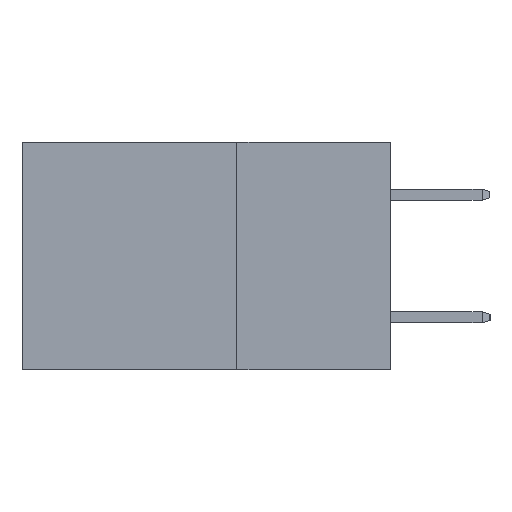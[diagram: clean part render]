
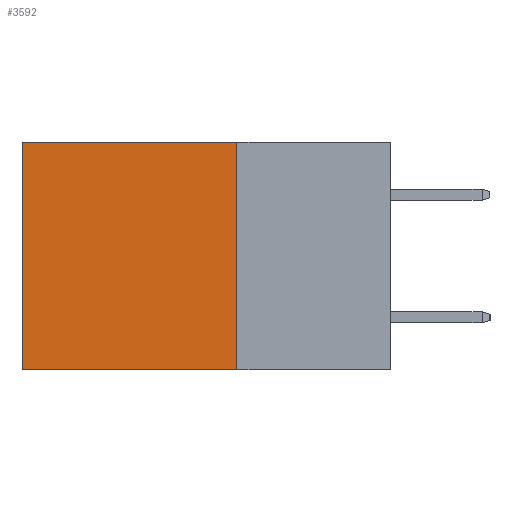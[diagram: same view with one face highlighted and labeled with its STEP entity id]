
A CAD part, left-side view. The second image highlights one B-rep face of the part: STEP entity #3592.
In plain terms, the highlighted planar face has unit normal (-1, 0, 0).
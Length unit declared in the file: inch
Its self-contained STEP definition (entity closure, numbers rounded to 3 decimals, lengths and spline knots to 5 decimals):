
#860 = ORIENTED_EDGE ( 'NONE', *, *, #4558, .F. ) ;
#1102 = VERTEX_POINT ( 'NONE', #10392 ) ;
#1399 = DIRECTION ( 'NONE',  ( 0., 0., -1. ) ) ;
#1477 = VERTEX_POINT ( 'NONE', #8669 ) ;
#1586 = ORIENTED_EDGE ( 'NONE', *, *, #10714, .T. ) ;
#1607 = VERTEX_POINT ( 'NONE', #12531 ) ;
#2351 = DIRECTION ( 'NONE',  ( 1., 0., 0. ) ) ;
#2871 = ORIENTED_EDGE ( 'NONE', *, *, #3994, .T. ) ;
#3326 = CARTESIAN_POINT ( 'NONE',  ( 0.2875, 0.25, 0. ) ) ;
#3592 = ADVANCED_FACE ( 'NONE', ( #5647 ), #9810, .F. ) ;
#3950 = LINE ( 'NONE', #3326, #10380 ) ;
#3994 = EDGE_CURVE ( 'NONE', #1607, #1477, #13299, .T. ) ;
#4436 = LINE ( 'NONE', #9249, #7094 ) ;
#4558 = EDGE_CURVE ( 'NONE', #1102, #9808, #4436, .T. ) ;
#5647 = FACE_OUTER_BOUND ( 'NONE', #9036, .T. ) ;
#7094 = VECTOR ( 'NONE', #1399, 39.37008 ) ;
#8139 = CARTESIAN_POINT ( 'NONE',  ( 0.2875, 0.25, -0.37 ) ) ;
#8602 = CARTESIAN_POINT ( 'NONE',  ( 0.2875, 0.25, 0. ) ) ;
#8669 = CARTESIAN_POINT ( 'NONE',  ( 0.2875, 0.6, -0.37 ) ) ;
#8884 = DIRECTION ( 'NONE',  ( 0., 0., -1. ) ) ;
#9036 = EDGE_LOOP ( 'NONE', ( #2871, #10672, #860, #1586 ) ) ;
#9249 = CARTESIAN_POINT ( 'NONE',  ( 0.2875, 0.25, 0. ) ) ;
#9670 = DIRECTION ( 'NONE',  ( 0., 1., 0. ) ) ;
#9713 = AXIS2_PLACEMENT_3D ( 'NONE', #8602, #2351, #12806 ) ;
#9808 = VERTEX_POINT ( 'NONE', #8139 ) ;
#9810 = PLANE ( 'NONE',  #9713 ) ;
#10051 = CARTESIAN_POINT ( 'NONE',  ( 0.2875, 0.25, -0.37 ) ) ;
#10380 = VECTOR ( 'NONE', #9670, 39.37008 ) ;
#10392 = CARTESIAN_POINT ( 'NONE',  ( 0.2875, 0.25, 0. ) ) ;
#10672 = ORIENTED_EDGE ( 'NONE', *, *, #12895, .F. ) ;
#10714 = EDGE_CURVE ( 'NONE', #1102, #1607, #3950, .T. ) ;
#10948 = DIRECTION ( 'NONE',  ( 0., 1., 0. ) ) ;
#11050 = VECTOR ( 'NONE', #8884, 39.37008 ) ;
#12303 = LINE ( 'NONE', #10051, #12455 ) ;
#12455 = VECTOR ( 'NONE', #10948, 39.37008 ) ;
#12531 = CARTESIAN_POINT ( 'NONE',  ( 0.2875, 0.6, 0. ) ) ;
#12806 = DIRECTION ( 'NONE',  ( 0., 0., -1. ) ) ;
#12895 = EDGE_CURVE ( 'NONE', #9808, #1477, #12303, .T. ) ;
#13127 = CARTESIAN_POINT ( 'NONE',  ( 0.2875, 0.6, 0. ) ) ;
#13299 = LINE ( 'NONE', #13127, #11050 ) ;
